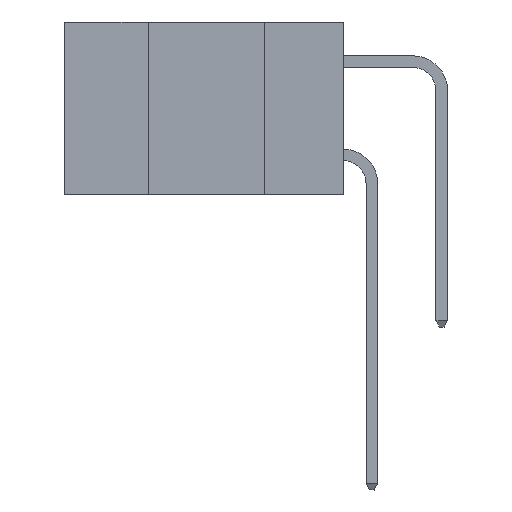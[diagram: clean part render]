
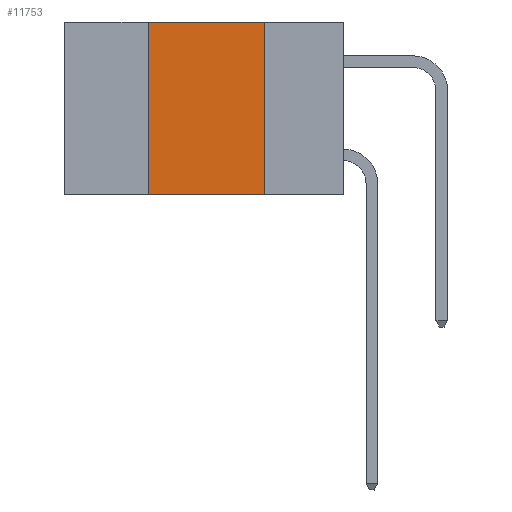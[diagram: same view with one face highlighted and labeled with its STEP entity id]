
A CAD part, left-side view. The second image highlights one B-rep face of the part: STEP entity #11753.
In plain terms, the highlighted planar face has unit normal (-1, 0, 0).
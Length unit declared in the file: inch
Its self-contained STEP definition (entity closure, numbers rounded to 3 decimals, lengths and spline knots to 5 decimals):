
#146 = DIRECTION ( 'NONE',  ( 1., 0., 0. ) ) ;
#1876 = CARTESIAN_POINT ( 'NONE',  ( 0., 0.17, -0.37 ) ) ;
#3968 = LINE ( 'NONE', #1876, #9644 ) ;
#4087 = VERTEX_POINT ( 'NONE', #14678 ) ;
#4128 = AXIS2_PLACEMENT_3D ( 'NONE', #10091, #146, #10356 ) ;
#6299 = ORIENTED_EDGE ( 'NONE', *, *, #22179, .T. ) ;
#6320 = VERTEX_POINT ( 'NONE', #17676 ) ;
#6860 = ORIENTED_EDGE ( 'NONE', *, *, #22560, .F. ) ;
#7210 = VECTOR ( 'NONE', #14416, 39.37008 ) ;
#7706 = CARTESIAN_POINT ( 'NONE',  ( 0., 0.6, 0. ) ) ;
#8909 = VECTOR ( 'NONE', #15721, 39.37008 ) ;
#9392 = CARTESIAN_POINT ( 'NONE',  ( 0., 0.6, -0.37 ) ) ;
#9644 = VECTOR ( 'NONE', #23930, 39.37008 ) ;
#10091 = CARTESIAN_POINT ( 'NONE',  ( 0., 0.6, 0. ) ) ;
#10356 = DIRECTION ( 'NONE',  ( 0., 0., -1. ) ) ;
#10852 = VERTEX_POINT ( 'NONE', #22536 ) ;
#11753 = ADVANCED_FACE ( 'NONE', ( #22316 ), #20346, .F. ) ;
#11773 = DIRECTION ( 'NONE',  ( 0., -1., 0. ) ) ;
#12006 = EDGE_LOOP ( 'NONE', ( #19418, #6860, #23871, #6299 ) ) ;
#12953 = VERTEX_POINT ( 'NONE', #19085 ) ;
#13467 = LINE ( 'NONE', #9392, #16481 ) ;
#14032 = LINE ( 'NONE', #24154, #7210 ) ;
#14416 = DIRECTION ( 'NONE',  ( 0., 0., 1. ) ) ;
#14678 = CARTESIAN_POINT ( 'NONE',  ( 0., 0.17, -0.37 ) ) ;
#15721 = DIRECTION ( 'NONE',  ( 0., -1., 0. ) ) ;
#15995 = EDGE_CURVE ( 'NONE', #12953, #4087, #3968, .T. ) ;
#16481 = VECTOR ( 'NONE', #11773, 39.37008 ) ;
#17676 = CARTESIAN_POINT ( 'NONE',  ( 0., 0.42, 0. ) ) ;
#19085 = CARTESIAN_POINT ( 'NONE',  ( 0., 0.17, 0. ) ) ;
#19418 = ORIENTED_EDGE ( 'NONE', *, *, #15995, .F. ) ;
#20346 = PLANE ( 'NONE',  #4128 ) ;
#21945 = EDGE_CURVE ( 'NONE', #10852, #6320, #14032, .T. ) ;
#22179 = EDGE_CURVE ( 'NONE', #10852, #4087, #13467, .T. ) ;
#22316 = FACE_OUTER_BOUND ( 'NONE', #12006, .T. ) ;
#22536 = CARTESIAN_POINT ( 'NONE',  ( 0., 0.42, -0.37 ) ) ;
#22560 = EDGE_CURVE ( 'NONE', #6320, #12953, #23618, .T. ) ;
#23618 = LINE ( 'NONE', #7706, #8909 ) ;
#23871 = ORIENTED_EDGE ( 'NONE', *, *, #21945, .F. ) ;
#23930 = DIRECTION ( 'NONE',  ( 0., 0., -1. ) ) ;
#24154 = CARTESIAN_POINT ( 'NONE',  ( 0., 0.42, -0.37 ) ) ;
